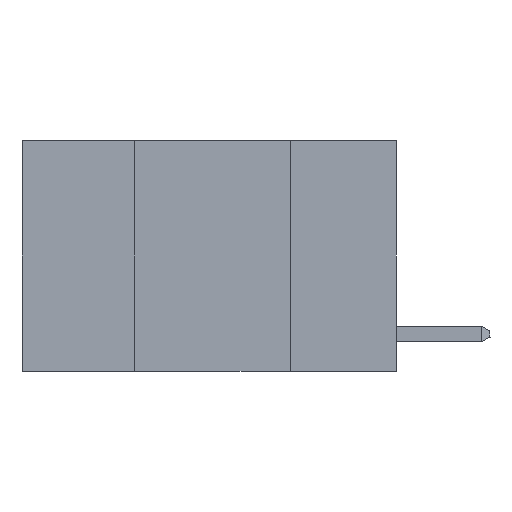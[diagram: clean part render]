
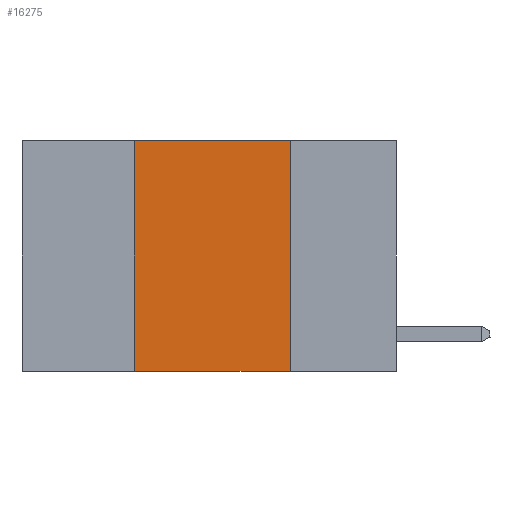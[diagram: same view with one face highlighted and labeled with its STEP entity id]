
A CAD part, left-side view. The second image highlights one B-rep face of the part: STEP entity #16275.
In plain terms, the highlighted planar face has unit normal (-1, 0, 0).
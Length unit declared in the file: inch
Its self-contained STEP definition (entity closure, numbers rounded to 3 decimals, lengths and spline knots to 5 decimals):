
#371 = LINE ( 'NONE', #4881, #21491 ) ;
#1054 = CARTESIAN_POINT ( 'NONE',  ( 0., 0.6, 0. ) ) ;
#2720 = VERTEX_POINT ( 'NONE', #5856 ) ;
#2909 = PLANE ( 'NONE',  #15255 ) ;
#2965 = EDGE_CURVE ( 'NONE', #13686, #2720, #371, .T. ) ;
#3369 = ORIENTED_EDGE ( 'NONE', *, *, #23668, .T. ) ;
#3646 = ORIENTED_EDGE ( 'NONE', *, *, #6814, .F. ) ;
#4050 = ORIENTED_EDGE ( 'NONE', *, *, #24776, .F. ) ;
#4881 = CARTESIAN_POINT ( 'NONE',  ( 0., 0.42, 0. ) ) ;
#5160 = LINE ( 'NONE', #1054, #24101 ) ;
#5669 = LINE ( 'NONE', #26684, #23284 ) ;
#5856 = CARTESIAN_POINT ( 'NONE',  ( 0., 0.42, 0. ) ) ;
#6141 = CARTESIAN_POINT ( 'NONE',  ( 0., 0.42, -0.37 ) ) ;
#6814 = EDGE_CURVE ( 'NONE', #2720, #25837, #5160, .T. ) ;
#8250 = VERTEX_POINT ( 'NONE', #17420 ) ;
#8550 = EDGE_LOOP ( 'NONE', ( #4050, #3646, #12645, #3369 ) ) ;
#9024 = DIRECTION ( 'NONE',  ( 0., -1., 0. ) ) ;
#10506 = CARTESIAN_POINT ( 'NONE',  ( 0., 0.17, 0. ) ) ;
#10617 = VECTOR ( 'NONE', #18051, 39.37008 ) ;
#11494 = CARTESIAN_POINT ( 'NONE',  ( 0., 0.17, 0. ) ) ;
#12645 = ORIENTED_EDGE ( 'NONE', *, *, #2965, .F. ) ;
#13686 = VERTEX_POINT ( 'NONE', #6141 ) ;
#15255 = AXIS2_PLACEMENT_3D ( 'NONE', #17600, #19548, #19824 ) ;
#16243 = DIRECTION ( 'NONE',  ( 0., -1., 0. ) ) ;
#16275 = ADVANCED_FACE ( 'NONE', ( #25720 ), #2909, .F. ) ;
#17420 = CARTESIAN_POINT ( 'NONE',  ( 0., 0.17, -0.37 ) ) ;
#17600 = CARTESIAN_POINT ( 'NONE',  ( 0., 0.6, 0. ) ) ;
#18051 = DIRECTION ( 'NONE',  ( 0., 0., -1. ) ) ;
#19548 = DIRECTION ( 'NONE',  ( 1., 0., 0. ) ) ;
#19824 = DIRECTION ( 'NONE',  ( 0., 0., -1. ) ) ;
#21491 = VECTOR ( 'NONE', #23567, 39.37008 ) ;
#23284 = VECTOR ( 'NONE', #16243, 39.37008 ) ;
#23567 = DIRECTION ( 'NONE',  ( 0., 0., 1. ) ) ;
#23668 = EDGE_CURVE ( 'NONE', #13686, #8250, #5669, .T. ) ;
#24101 = VECTOR ( 'NONE', #9024, 39.37008 ) ;
#24381 = LINE ( 'NONE', #11494, #10617 ) ;
#24776 = EDGE_CURVE ( 'NONE', #25837, #8250, #24381, .T. ) ;
#25720 = FACE_OUTER_BOUND ( 'NONE', #8550, .T. ) ;
#25837 = VERTEX_POINT ( 'NONE', #10506 ) ;
#26684 = CARTESIAN_POINT ( 'NONE',  ( 0., 0.6, -0.37 ) ) ;
